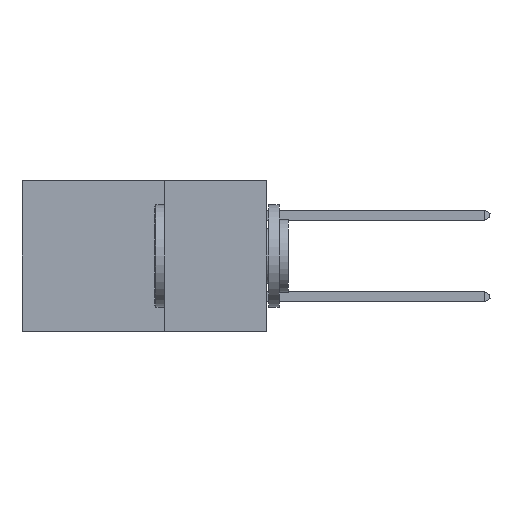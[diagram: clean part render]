
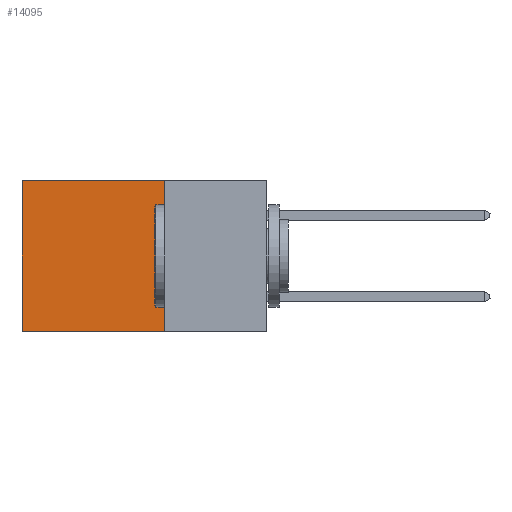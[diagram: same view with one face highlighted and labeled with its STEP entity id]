
A CAD part, left-side view. The second image highlights one B-rep face of the part: STEP entity #14095.
In plain terms, the highlighted planar face has unit normal (-1, 0, 0).
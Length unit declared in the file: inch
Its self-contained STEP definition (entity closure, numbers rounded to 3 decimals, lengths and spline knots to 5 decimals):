
#164 = VECTOR ( 'NONE', #599, 39.37008 ) ;
#512 = CARTESIAN_POINT ( 'NONE',  ( 0.2875, 0.25, 0. ) ) ;
#599 = DIRECTION ( 'NONE',  ( 0., 1., 0. ) ) ;
#2100 = DIRECTION ( 'NONE',  ( 0., 0., -1. ) ) ;
#2513 = DIRECTION ( 'NONE',  ( 0., 1., 0. ) ) ;
#2723 = DIRECTION ( 'NONE',  ( 1., 0., 0. ) ) ;
#6648 = VECTOR ( 'NONE', #2100, 39.37008 ) ;
#6767 = ORIENTED_EDGE ( 'NONE', *, *, #14653, .T. ) ;
#6905 = EDGE_CURVE ( 'NONE', #7615, #13939, #19942, .T. ) ;
#7615 = VERTEX_POINT ( 'NONE', #7732 ) ;
#7732 = CARTESIAN_POINT ( 'NONE',  ( 0.2875, 0.25, -0.37 ) ) ;
#8076 = FACE_OUTER_BOUND ( 'NONE', #18802, .T. ) ;
#9295 = LINE ( 'NONE', #512, #164 ) ;
#9333 = DIRECTION ( 'NONE',  ( 0., 0., -1. ) ) ;
#9738 = ORIENTED_EDGE ( 'NONE', *, *, #6905, .F. ) ;
#9942 = CARTESIAN_POINT ( 'NONE',  ( 0.2875, 0.25, 0. ) ) ;
#12041 = VECTOR ( 'NONE', #2513, 39.37008 ) ;
#12531 = DIRECTION ( 'NONE',  ( 0., 0., -1. ) ) ;
#12959 = VERTEX_POINT ( 'NONE', #13602 ) ;
#13514 = ORIENTED_EDGE ( 'NONE', *, *, #24955, .F. ) ;
#13602 = CARTESIAN_POINT ( 'NONE',  ( 0.2875, 0.6, 0. ) ) ;
#13826 = CARTESIAN_POINT ( 'NONE',  ( 0.2875, 0.6, -0.37 ) ) ;
#13939 = VERTEX_POINT ( 'NONE', #13826 ) ;
#14013 = AXIS2_PLACEMENT_3D ( 'NONE', #22208, #2723, #12531 ) ;
#14095 = ADVANCED_FACE ( 'NONE', ( #8076 ), #20256, .F. ) ;
#14177 = CARTESIAN_POINT ( 'NONE',  ( 0.2875, 0.25, -0.37 ) ) ;
#14653 = EDGE_CURVE ( 'NONE', #22477, #12959, #9295, .T. ) ;
#15695 = ORIENTED_EDGE ( 'NONE', *, *, #20785, .T. ) ;
#18802 = EDGE_LOOP ( 'NONE', ( #15695, #9738, #13514, #6767 ) ) ;
#19756 = LINE ( 'NONE', #24821, #21879 ) ;
#19942 = LINE ( 'NONE', #14177, #12041 ) ;
#20256 = PLANE ( 'NONE',  #14013 ) ;
#20785 = EDGE_CURVE ( 'NONE', #12959, #13939, #19756, .T. ) ;
#21693 = CARTESIAN_POINT ( 'NONE',  ( 0.2875, 0.25, 0. ) ) ;
#21879 = VECTOR ( 'NONE', #9333, 39.37008 ) ;
#22208 = CARTESIAN_POINT ( 'NONE',  ( 0.2875, 0.25, 0. ) ) ;
#22477 = VERTEX_POINT ( 'NONE', #21693 ) ;
#24821 = CARTESIAN_POINT ( 'NONE',  ( 0.2875, 0.6, 0. ) ) ;
#24940 = LINE ( 'NONE', #9942, #6648 ) ;
#24955 = EDGE_CURVE ( 'NONE', #22477, #7615, #24940, .T. ) ;
